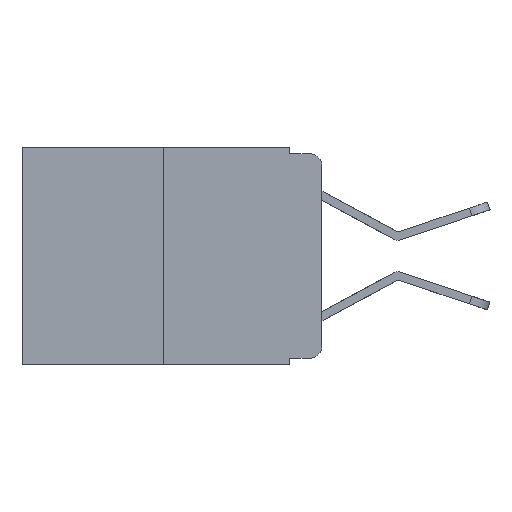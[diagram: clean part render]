
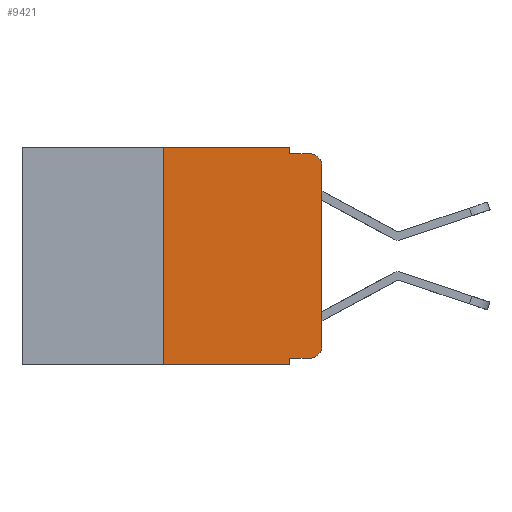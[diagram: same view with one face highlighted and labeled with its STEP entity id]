
A CAD part, left-side view. The second image highlights one B-rep face of the part: STEP entity #9421.
In plain terms, the highlighted planar face has unit normal (-1, 0, 0).
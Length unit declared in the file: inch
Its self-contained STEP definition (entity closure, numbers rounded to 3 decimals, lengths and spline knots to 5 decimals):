
#4 = ORIENTED_EDGE ( 'NONE', *, *, #6310, .T. ) ;
#158 = DIRECTION ( 'NONE',  ( 1., 0., 0. ) ) ;
#223 = VERTEX_POINT ( 'NONE', #18357 ) ;
#271 = VECTOR ( 'NONE', #12407, 39.37008 ) ;
#526 = CARTESIAN_POINT ( 'NONE',  ( 0., 0.25, 0. ) ) ;
#539 = VECTOR ( 'NONE', #5861, 39.37008 ) ;
#1234 = DIRECTION ( 'NONE',  ( -1., 0., 0. ) ) ;
#1731 = EDGE_CURVE ( 'NONE', #4769, #18963, #16024, .T. ) ;
#2451 = LINE ( 'NONE', #526, #10130 ) ;
#2554 = ORIENTED_EDGE ( 'NONE', *, *, #17430, .F. ) ;
#2616 = LINE ( 'NONE', #11532, #17792 ) ;
#2815 = EDGE_CURVE ( 'NONE', #18048, #4769, #10775, .T. ) ;
#3273 = ORIENTED_EDGE ( 'NONE', *, *, #1731, .F. ) ;
#3410 = PLANE ( 'NONE',  #7240 ) ;
#3626 = ORIENTED_EDGE ( 'NONE', *, *, #19492, .T. ) ;
#3807 = DIRECTION ( 'NONE',  ( 0., 0., 1. ) ) ;
#4564 = CARTESIAN_POINT ( 'NONE',  ( 0., 0.051, 0. ) ) ;
#4744 = CIRCLE ( 'NONE', #8906, 0.02 ) ;
#4769 = VERTEX_POINT ( 'NONE', #15734 ) ;
#4851 = EDGE_CURVE ( 'NONE', #6412, #6250, #2616, .T. ) ;
#4957 = ORIENTED_EDGE ( 'NONE', *, *, #18428, .F. ) ;
#5167 = DIRECTION ( 'NONE',  ( 0., 0., -1. ) ) ;
#5190 = CARTESIAN_POINT ( 'NONE',  ( 0., 0., -0.03 ) ) ;
#5194 = VECTOR ( 'NONE', #17556, 39.37008 ) ;
#5688 = AXIS2_PLACEMENT_3D ( 'NONE', #6613, #15549, #6474 ) ;
#5861 = DIRECTION ( 'NONE',  ( 0., -1., 0. ) ) ;
#5936 = EDGE_CURVE ( 'NONE', #6250, #18963, #7877, .T. ) ;
#6250 = VERTEX_POINT ( 'NONE', #5190 ) ;
#6310 = EDGE_CURVE ( 'NONE', #9650, #223, #13766, .T. ) ;
#6412 = VERTEX_POINT ( 'NONE', #11183 ) ;
#6424 = ORIENTED_EDGE ( 'NONE', *, *, #4851, .T. ) ;
#6449 = CARTESIAN_POINT ( 'NONE',  ( 0., 0.051, -0.01 ) ) ;
#6474 = DIRECTION ( 'NONE',  ( 0., 0., -1. ) ) ;
#6613 = CARTESIAN_POINT ( 'NONE',  ( 0., 0.02, -0.03 ) ) ;
#6765 = VECTOR ( 'NONE', #5167, 39.37008 ) ;
#7105 = CARTESIAN_POINT ( 'NONE',  ( 0., 0.051, -0.333 ) ) ;
#7240 = AXIS2_PLACEMENT_3D ( 'NONE', #17060, #158, #11099 ) ;
#7877 = CIRCLE ( 'NONE', #5688, 0.02 ) ;
#8007 = VECTOR ( 'NONE', #8807, 39.37008 ) ;
#8777 = EDGE_LOOP ( 'NONE', ( #6424, #10449, #3273, #9291, #14241, #2554, #12583, #4957, #4, #3626 ) ) ;
#8807 = DIRECTION ( 'NONE',  ( 0., -1., 0. ) ) ;
#8906 = AXIS2_PLACEMENT_3D ( 'NONE', #10519, #1234, #12048 ) ;
#9072 = VERTEX_POINT ( 'NONE', #13131 ) ;
#9291 = ORIENTED_EDGE ( 'NONE', *, *, #2815, .F. ) ;
#9421 = ADVANCED_FACE ( 'NONE', ( #19312 ), #3410, .F. ) ;
#9650 = VERTEX_POINT ( 'NONE', #19128 ) ;
#9763 = EDGE_CURVE ( 'NONE', #9072, #18048, #18150, .T. ) ;
#10130 = VECTOR ( 'NONE', #3807, 39.37008 ) ;
#10449 = ORIENTED_EDGE ( 'NONE', *, *, #5936, .T. ) ;
#10519 = CARTESIAN_POINT ( 'NONE',  ( 0., 0.02, -0.313 ) ) ;
#10775 = LINE ( 'NONE', #4564, #6765 ) ;
#11099 = DIRECTION ( 'NONE',  ( 0., 0., -1. ) ) ;
#11183 = CARTESIAN_POINT ( 'NONE',  ( 0., 0., -0.313 ) ) ;
#11532 = CARTESIAN_POINT ( 'NONE',  ( 0., 0., 0. ) ) ;
#12048 = DIRECTION ( 'NONE',  ( 0., 0., -1. ) ) ;
#12407 = DIRECTION ( 'NONE',  ( 0., 0., -1. ) ) ;
#12583 = ORIENTED_EDGE ( 'NONE', *, *, #18218, .T. ) ;
#12681 = LINE ( 'NONE', #16853, #271 ) ;
#13131 = CARTESIAN_POINT ( 'NONE',  ( 0., 0.25, 0. ) ) ;
#13404 = CARTESIAN_POINT ( 'NONE',  ( 0., 0.473, 0. ) ) ;
#13711 = VECTOR ( 'NONE', #17904, 39.37008 ) ;
#13759 = DIRECTION ( 'NONE',  ( 0., 0., 1. ) ) ;
#13766 = LINE ( 'NONE', #7105, #5194 ) ;
#14241 = ORIENTED_EDGE ( 'NONE', *, *, #9763, .F. ) ;
#14707 = VERTEX_POINT ( 'NONE', #19044 ) ;
#15549 = DIRECTION ( 'NONE',  ( -1., 0., 0. ) ) ;
#15734 = CARTESIAN_POINT ( 'NONE',  ( 0., 0.051, -0.01 ) ) ;
#15892 = CARTESIAN_POINT ( 'NONE',  ( 0., 0.051, 0. ) ) ;
#16024 = LINE ( 'NONE', #6449, #8007 ) ;
#16853 = CARTESIAN_POINT ( 'NONE',  ( 0., 0.051, 0. ) ) ;
#16901 = LINE ( 'NONE', #17856, #539 ) ;
#17060 = CARTESIAN_POINT ( 'NONE',  ( 0., 0.473, 0. ) ) ;
#17430 = EDGE_CURVE ( 'NONE', #18983, #9072, #2451, .T. ) ;
#17556 = DIRECTION ( 'NONE',  ( 0., -1., 0. ) ) ;
#17792 = VECTOR ( 'NONE', #13759, 39.37008 ) ;
#17856 = CARTESIAN_POINT ( 'NONE',  ( 0., 0.473, -0.343 ) ) ;
#17904 = DIRECTION ( 'NONE',  ( 0., -1., 0. ) ) ;
#18048 = VERTEX_POINT ( 'NONE', #15892 ) ;
#18150 = LINE ( 'NONE', #13404, #13711 ) ;
#18218 = EDGE_CURVE ( 'NONE', #18983, #14707, #16901, .T. ) ;
#18280 = CARTESIAN_POINT ( 'NONE',  ( 0., 0.25, -0.343 ) ) ;
#18357 = CARTESIAN_POINT ( 'NONE',  ( 0., 0.02, -0.333 ) ) ;
#18428 = EDGE_CURVE ( 'NONE', #9650, #14707, #12681, .T. ) ;
#18963 = VERTEX_POINT ( 'NONE', #19688 ) ;
#18983 = VERTEX_POINT ( 'NONE', #18280 ) ;
#19044 = CARTESIAN_POINT ( 'NONE',  ( 0., 0.051, -0.343 ) ) ;
#19128 = CARTESIAN_POINT ( 'NONE',  ( 0., 0.051, -0.333 ) ) ;
#19312 = FACE_OUTER_BOUND ( 'NONE', #8777, .T. ) ;
#19492 = EDGE_CURVE ( 'NONE', #223, #6412, #4744, .T. ) ;
#19688 = CARTESIAN_POINT ( 'NONE',  ( 0., 0.02, -0.01 ) ) ;
